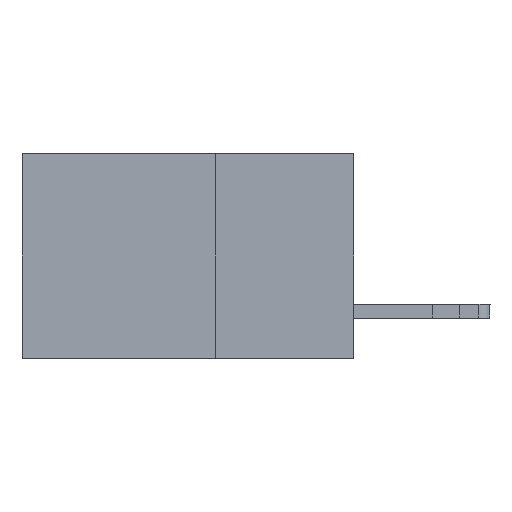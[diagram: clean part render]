
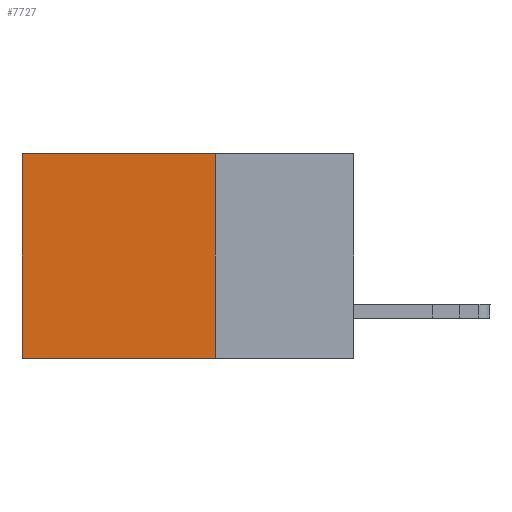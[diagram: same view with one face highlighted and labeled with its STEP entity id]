
A CAD part, left-side view. The second image highlights one B-rep face of the part: STEP entity #7727.
In plain terms, the highlighted planar face has unit normal (-1, 0, 0).
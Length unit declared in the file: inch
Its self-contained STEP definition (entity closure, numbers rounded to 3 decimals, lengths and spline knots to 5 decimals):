
#231 = VERTEX_POINT ( 'NONE', #13267 ) ;
#997 = CARTESIAN_POINT ( 'NONE',  ( 0.2875, 0.25, -0.37 ) ) ;
#1067 = PLANE ( 'NONE',  #9061 ) ;
#1840 = CARTESIAN_POINT ( 'NONE',  ( 0.2875, 0.25, -0.37 ) ) ;
#2634 = LINE ( 'NONE', #11369, #4727 ) ;
#3480 = ORIENTED_EDGE ( 'NONE', *, *, #13179, .F. ) ;
#4042 = VERTEX_POINT ( 'NONE', #997 ) ;
#4727 = VECTOR ( 'NONE', #5163, 39.37008 ) ;
#4798 = VECTOR ( 'NONE', #9206, 39.37008 ) ;
#4834 = DIRECTION ( 'NONE',  ( 0., 0., -1. ) ) ;
#4868 = ORIENTED_EDGE ( 'NONE', *, *, #5000, .F. ) ;
#5000 = EDGE_CURVE ( 'NONE', #4042, #5950, #12798, .T. ) ;
#5163 = DIRECTION ( 'NONE',  ( 0., 1., 0. ) ) ;
#5543 = CARTESIAN_POINT ( 'NONE',  ( 0.2875, 0.25, 0. ) ) ;
#5950 = VERTEX_POINT ( 'NONE', #11303 ) ;
#7374 = EDGE_CURVE ( 'NONE', #231, #14215, #2634, .T. ) ;
#7727 = ADVANCED_FACE ( 'NONE', ( #13297 ), #1067, .F. ) ;
#7769 = EDGE_CURVE ( 'NONE', #14215, #5950, #8417, .T. ) ;
#8001 = LINE ( 'NONE', #5543, #11313 ) ;
#8031 = VECTOR ( 'NONE', #4834, 39.37008 ) ;
#8417 = LINE ( 'NONE', #12285, #8031 ) ;
#9061 = AXIS2_PLACEMENT_3D ( 'NONE', #14742, #9620, #9563 ) ;
#9206 = DIRECTION ( 'NONE',  ( 0., 1., 0. ) ) ;
#9405 = DIRECTION ( 'NONE',  ( 0., 0., -1. ) ) ;
#9563 = DIRECTION ( 'NONE',  ( 0., 0., -1. ) ) ;
#9620 = DIRECTION ( 'NONE',  ( 1., 0., 0. ) ) ;
#9903 = EDGE_LOOP ( 'NONE', ( #15470, #4868, #3480, #10360 ) ) ;
#10360 = ORIENTED_EDGE ( 'NONE', *, *, #7374, .T. ) ;
#11018 = CARTESIAN_POINT ( 'NONE',  ( 0.2875, 0.6, 0. ) ) ;
#11303 = CARTESIAN_POINT ( 'NONE',  ( 0.2875, 0.6, -0.37 ) ) ;
#11313 = VECTOR ( 'NONE', #9405, 39.37008 ) ;
#11369 = CARTESIAN_POINT ( 'NONE',  ( 0.2875, 0.25, 0. ) ) ;
#12285 = CARTESIAN_POINT ( 'NONE',  ( 0.2875, 0.6, 0. ) ) ;
#12798 = LINE ( 'NONE', #1840, #4798 ) ;
#13179 = EDGE_CURVE ( 'NONE', #231, #4042, #8001, .T. ) ;
#13267 = CARTESIAN_POINT ( 'NONE',  ( 0.2875, 0.25, 0. ) ) ;
#13297 = FACE_OUTER_BOUND ( 'NONE', #9903, .T. ) ;
#14215 = VERTEX_POINT ( 'NONE', #11018 ) ;
#14742 = CARTESIAN_POINT ( 'NONE',  ( 0.2875, 0.25, 0. ) ) ;
#15470 = ORIENTED_EDGE ( 'NONE', *, *, #7769, .T. ) ;
